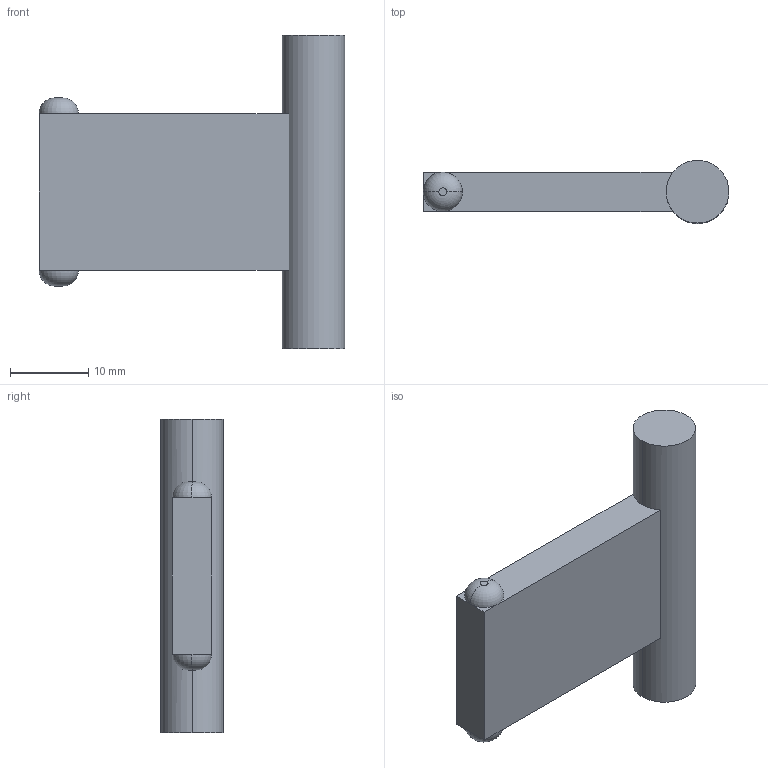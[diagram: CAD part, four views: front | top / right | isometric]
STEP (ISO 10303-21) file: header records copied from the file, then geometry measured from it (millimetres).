
FILE_DESCRIPTION (( 'STEP AP203' ), '1' );
FILE_NAME ('follower.STEP', '2013-09-09T02:51:01', ( '' ), ( '' ), 'SwSTEP 2.0', 'SolidWorks 2013', '' );
FILE_SCHEMA (( 'CONFIG_CONTROL_DESIGN' ));
Length unit declared in the file: millimetre
Products named in the file (1): follower
Bounding box: 39 x 8 x 40 mm (x, y, z)
Volume: 5194.8 mm3; surface area: 2718 mm2
Topology: 1 solids, 1 shells, 19 faces, 43 edges, 26 vertices
Faces by surface type: plane 13, torus 4, cylinder 2
Entity records: 614 total; most frequent: DIRECTION 107, CARTESIAN_POINT 89, ORIENTED_EDGE 86, AXIS2_PLACEMENT_3D 44, EDGE_CURVE 43, VERTEX_POINT 26, CIRCLE 24, FACE_OUTER_BOUND 19
